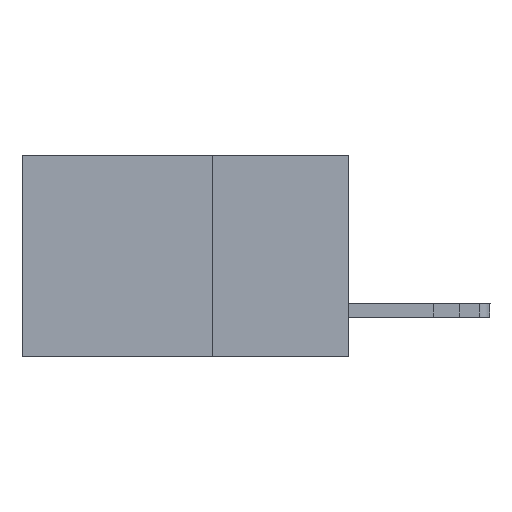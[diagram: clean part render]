
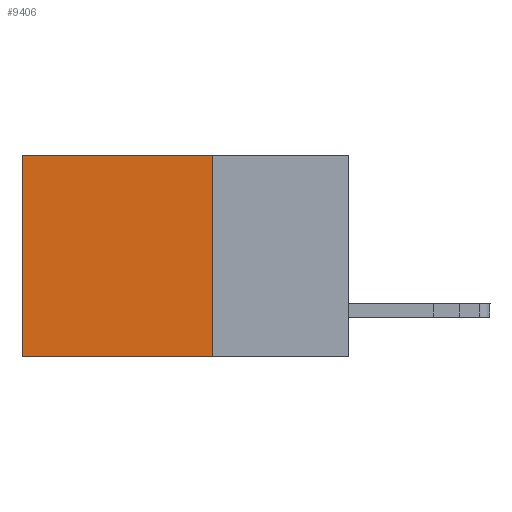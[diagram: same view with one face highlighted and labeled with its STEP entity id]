
A CAD part, left-side view. The second image highlights one B-rep face of the part: STEP entity #9406.
In plain terms, the highlighted planar face has unit normal (-1, 0, 0).
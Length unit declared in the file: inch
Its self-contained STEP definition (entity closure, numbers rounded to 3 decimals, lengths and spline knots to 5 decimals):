
#111 = VECTOR ( 'NONE', #14691, 39.37008 ) ;
#689 = DIRECTION ( 'NONE',  ( 0., 0., -1. ) ) ;
#1027 = VECTOR ( 'NONE', #1900, 39.37008 ) ;
#1142 = VERTEX_POINT ( 'NONE', #7137 ) ;
#1900 = DIRECTION ( 'NONE',  ( 0., 0., -1. ) ) ;
#2206 = LINE ( 'NONE', #16177, #111 ) ;
#2275 = VERTEX_POINT ( 'NONE', #9882 ) ;
#3168 = EDGE_CURVE ( 'NONE', #1142, #5202, #12122, .T. ) ;
#3352 = ORIENTED_EDGE ( 'NONE', *, *, #10205, .T. ) ;
#4342 = DIRECTION ( 'NONE',  ( 0., 1., 0. ) ) ;
#5202 = VERTEX_POINT ( 'NONE', #19412 ) ;
#5613 = ORIENTED_EDGE ( 'NONE', *, *, #16482, .F. ) ;
#6720 = LINE ( 'NONE', #8291, #18108 ) ;
#6776 = DIRECTION ( 'NONE',  ( 1., 0., 0. ) ) ;
#7137 = CARTESIAN_POINT ( 'NONE',  ( 0.298, 0.25, -0.37 ) ) ;
#7369 = CARTESIAN_POINT ( 'NONE',  ( 0.298, 0.25, -0.37 ) ) ;
#8291 = CARTESIAN_POINT ( 'NONE',  ( 0.298, 0.25, 0. ) ) ;
#8494 = LINE ( 'NONE', #9964, #1027 ) ;
#9090 = VERTEX_POINT ( 'NONE', #15121 ) ;
#9200 = ORIENTED_EDGE ( 'NONE', *, *, #18886, .T. ) ;
#9406 = ADVANCED_FACE ( 'NONE', ( #15066 ), #10237, .F. ) ;
#9882 = CARTESIAN_POINT ( 'NONE',  ( 0.298, 0.6, 0. ) ) ;
#9964 = CARTESIAN_POINT ( 'NONE',  ( 0.298, 0.25, 0. ) ) ;
#10205 = EDGE_CURVE ( 'NONE', #9090, #2275, #6720, .T. ) ;
#10237 = PLANE ( 'NONE',  #20434 ) ;
#11395 = CARTESIAN_POINT ( 'NONE',  ( 0.298, 0.25, 0. ) ) ;
#11938 = EDGE_LOOP ( 'NONE', ( #9200, #20393, #5613, #3352 ) ) ;
#12122 = LINE ( 'NONE', #7369, #15457 ) ;
#14691 = DIRECTION ( 'NONE',  ( 0., 0., -1. ) ) ;
#15066 = FACE_OUTER_BOUND ( 'NONE', #11938, .T. ) ;
#15121 = CARTESIAN_POINT ( 'NONE',  ( 0.298, 0.25, 0. ) ) ;
#15457 = VECTOR ( 'NONE', #4342, 39.37008 ) ;
#16177 = CARTESIAN_POINT ( 'NONE',  ( 0.298, 0.6, 0. ) ) ;
#16199 = DIRECTION ( 'NONE',  ( 0., 1., 0. ) ) ;
#16482 = EDGE_CURVE ( 'NONE', #9090, #1142, #8494, .T. ) ;
#18108 = VECTOR ( 'NONE', #16199, 39.37008 ) ;
#18886 = EDGE_CURVE ( 'NONE', #2275, #5202, #2206, .T. ) ;
#19412 = CARTESIAN_POINT ( 'NONE',  ( 0.298, 0.6, -0.37 ) ) ;
#20393 = ORIENTED_EDGE ( 'NONE', *, *, #3168, .F. ) ;
#20434 = AXIS2_PLACEMENT_3D ( 'NONE', #11395, #6776, #689 ) ;
